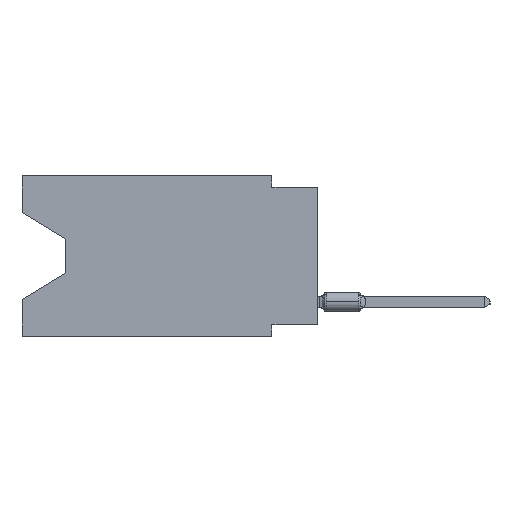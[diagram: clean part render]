
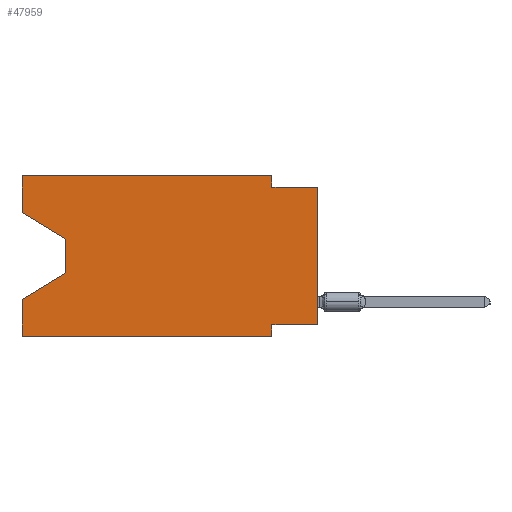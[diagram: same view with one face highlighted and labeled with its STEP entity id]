
A CAD part, left-side view. The second image highlights one B-rep face of the part: STEP entity #47959.
In plain terms, the highlighted planar face has unit normal (-1, 0, 0).
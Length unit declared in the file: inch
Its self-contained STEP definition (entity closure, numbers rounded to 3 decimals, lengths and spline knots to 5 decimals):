
#193 = LINE ( 'NONE', #41502, #43727 ) ;
#1086 = CARTESIAN_POINT ( 'NONE',  ( 0., 0.1, -0.325 ) ) ;
#1662 = EDGE_CURVE ( 'NONE', #44634, #39358, #8237, .T. ) ;
#1699 = ORIENTED_EDGE ( 'NONE', *, *, #1662, .F. ) ;
#5048 = VECTOR ( 'NONE', #38399, 39.37008 ) ;
#6948 = PLANE ( 'NONE',  #66461 ) ;
#7233 = CARTESIAN_POINT ( 'NONE',  ( 0., 0.1, -0.35 ) ) ;
#8237 = LINE ( 'NONE', #35169, #15306 ) ;
#8245 = CARTESIAN_POINT ( 'NONE',  ( 0., 0., 0. ) ) ;
#8708 = CARTESIAN_POINT ( 'NONE',  ( 0., 0.645, -0.08025 ) ) ;
#11009 = DIRECTION ( 'NONE',  ( 0., 0., -1. ) ) ;
#11106 = VERTEX_POINT ( 'NONE', #8708 ) ;
#11544 = DIRECTION ( 'NONE',  ( 0., 0.855, -0.519 ) ) ;
#11688 = VERTEX_POINT ( 'NONE', #55358 ) ;
#12210 = FACE_OUTER_BOUND ( 'NONE', #42204, .T. ) ;
#15266 = DIRECTION ( 'NONE',  ( 0., 0., -1. ) ) ;
#15306 = VECTOR ( 'NONE', #46365, 39.37008 ) ;
#16614 = VERTEX_POINT ( 'NONE', #1086 ) ;
#17595 = VECTOR ( 'NONE', #21850, 39.37008 ) ;
#18417 = LINE ( 'NONE', #8245, #66617 ) ;
#19380 = CARTESIAN_POINT ( 'NONE',  ( 0., 0.1, -0.025 ) ) ;
#20049 = VERTEX_POINT ( 'NONE', #58505 ) ;
#20349 = VERTEX_POINT ( 'NONE', #51467 ) ;
#21512 = CARTESIAN_POINT ( 'NONE',  ( 0., 0.645, 0. ) ) ;
#21850 = DIRECTION ( 'NONE',  ( 0., 0., 1. ) ) ;
#22328 = CARTESIAN_POINT ( 'NONE',  ( 0., 0., -0.325 ) ) ;
#23044 = DIRECTION ( 'NONE',  ( 1., 0., 0. ) ) ;
#23135 = CARTESIAN_POINT ( 'NONE',  ( 0., 0.645, -0.35 ) ) ;
#23706 = EDGE_CURVE ( 'NONE', #39358, #31492, #44220, .T. ) ;
#23986 = CARTESIAN_POINT ( 'NONE',  ( 0., 0.645, -0.08025 ) ) ;
#24188 = ORIENTED_EDGE ( 'NONE', *, *, #49521, .T. ) ;
#24286 = EDGE_CURVE ( 'NONE', #65336, #20349, #50383, .T. ) ;
#24344 = LINE ( 'NONE', #35849, #36367 ) ;
#24945 = ORIENTED_EDGE ( 'NONE', *, *, #31799, .F. ) ;
#27012 = CARTESIAN_POINT ( 'NONE',  ( 0., 0.55, -0.138 ) ) ;
#27184 = EDGE_CURVE ( 'NONE', #20049, #11688, #38129, .T. ) ;
#27426 = ORIENTED_EDGE ( 'NONE', *, *, #64969, .F. ) ;
#27688 = VERTEX_POINT ( 'NONE', #27012 ) ;
#28271 = CARTESIAN_POINT ( 'NONE',  ( 0., 0.645, 0. ) ) ;
#28664 = ORIENTED_EDGE ( 'NONE', *, *, #58988, .T. ) ;
#29293 = VECTOR ( 'NONE', #11544, 39.37008 ) ;
#30680 = ORIENTED_EDGE ( 'NONE', *, *, #48420, .F. ) ;
#31492 = VERTEX_POINT ( 'NONE', #19380 ) ;
#31799 = EDGE_CURVE ( 'NONE', #31492, #53319, #38565, .T. ) ;
#31977 = LINE ( 'NONE', #21512, #17595 ) ;
#32711 = VECTOR ( 'NONE', #43818, 39.37008 ) ;
#32771 = VERTEX_POINT ( 'NONE', #64544 ) ;
#33618 = DIRECTION ( 'NONE',  ( 0., -1., 0. ) ) ;
#33987 = VECTOR ( 'NONE', #65604, 39.37008 ) ;
#34493 = DIRECTION ( 'NONE',  ( 0., 0., 1. ) ) ;
#35124 = CARTESIAN_POINT ( 'NONE',  ( 0., 0.645, 0. ) ) ;
#35169 = CARTESIAN_POINT ( 'NONE',  ( 0., 0.645, 0. ) ) ;
#35849 = CARTESIAN_POINT ( 'NONE',  ( 0., 0.645, 0. ) ) ;
#36367 = VECTOR ( 'NONE', #45674, 39.37008 ) ;
#37210 = ORIENTED_EDGE ( 'NONE', *, *, #23706, .F. ) ;
#37277 = CARTESIAN_POINT ( 'NONE',  ( 0., 0.645, -0.35 ) ) ;
#38129 = LINE ( 'NONE', #64357, #29293 ) ;
#38399 = DIRECTION ( 'NONE',  ( 0., 1., 0. ) ) ;
#38565 = LINE ( 'NONE', #64450, #32711 ) ;
#38654 = ORIENTED_EDGE ( 'NONE', *, *, #56511, .F. ) ;
#39358 = VERTEX_POINT ( 'NONE', #50323 ) ;
#40774 = ORIENTED_EDGE ( 'NONE', *, *, #24286, .T. ) ;
#41502 = CARTESIAN_POINT ( 'NONE',  ( 0., 0.55, -0.138 ) ) ;
#42204 = EDGE_LOOP ( 'NONE', ( #67073, #28664, #67995, #49190, #40774, #38654, #27426, #24188, #24945, #37210, #1699, #30680 ) ) ;
#43727 = VECTOR ( 'NONE', #15266, 39.37008 ) ;
#43818 = DIRECTION ( 'NONE',  ( 0., -1., 0. ) ) ;
#44210 = CARTESIAN_POINT ( 'NONE',  ( 0., 0., -0.025 ) ) ;
#44220 = LINE ( 'NONE', #58909, #61406 ) ;
#44634 = VERTEX_POINT ( 'NONE', #35124 ) ;
#45674 = DIRECTION ( 'NONE',  ( 0., 0., 1. ) ) ;
#46365 = DIRECTION ( 'NONE',  ( 0., -1., 0. ) ) ;
#47026 = EDGE_CURVE ( 'NONE', #11106, #27688, #54436, .T. ) ;
#47959 = ADVANCED_FACE ( 'NONE', ( #12210 ), #6948, .F. ) ;
#48055 = VECTOR ( 'NONE', #33618, 39.37008 ) ;
#48420 = EDGE_CURVE ( 'NONE', #11106, #44634, #24344, .T. ) ;
#48906 = LINE ( 'NONE', #22328, #5048 ) ;
#49190 = ORIENTED_EDGE ( 'NONE', *, *, #67798, .F. ) ;
#49521 = EDGE_CURVE ( 'NONE', #32771, #53319, #18417, .T. ) ;
#49563 = DIRECTION ( 'NONE',  ( 0., 0., -1. ) ) ;
#50323 = CARTESIAN_POINT ( 'NONE',  ( 0., 0.1, 0. ) ) ;
#50383 = LINE ( 'NONE', #23135, #48055 ) ;
#51467 = CARTESIAN_POINT ( 'NONE',  ( 0., 0.1, -0.35 ) ) ;
#53319 = VERTEX_POINT ( 'NONE', #44210 ) ;
#54436 = LINE ( 'NONE', #23986, #33987 ) ;
#55358 = CARTESIAN_POINT ( 'NONE',  ( 0., 0.645, -0.26975 ) ) ;
#56511 = EDGE_CURVE ( 'NONE', #16614, #20349, #60390, .T. ) ;
#58505 = CARTESIAN_POINT ( 'NONE',  ( 0., 0.55, -0.212 ) ) ;
#58909 = CARTESIAN_POINT ( 'NONE',  ( 0., 0.1, 0. ) ) ;
#58988 = EDGE_CURVE ( 'NONE', #27688, #20049, #193, .T. ) ;
#60390 = LINE ( 'NONE', #7233, #63577 ) ;
#61406 = VECTOR ( 'NONE', #11009, 39.37008 ) ;
#63577 = VECTOR ( 'NONE', #49563, 39.37008 ) ;
#64357 = CARTESIAN_POINT ( 'NONE',  ( 0., 0.55, -0.212 ) ) ;
#64450 = CARTESIAN_POINT ( 'NONE',  ( 0., 0., -0.025 ) ) ;
#64544 = CARTESIAN_POINT ( 'NONE',  ( 0., 0., -0.325 ) ) ;
#64969 = EDGE_CURVE ( 'NONE', #32771, #16614, #48906, .T. ) ;
#65336 = VERTEX_POINT ( 'NONE', #37277 ) ;
#65604 = DIRECTION ( 'NONE',  ( 0., -0.855, -0.519 ) ) ;
#65693 = DIRECTION ( 'NONE',  ( 0., 0., -1. ) ) ;
#66461 = AXIS2_PLACEMENT_3D ( 'NONE', #28271, #23044, #65693 ) ;
#66617 = VECTOR ( 'NONE', #34493, 39.37008 ) ;
#67073 = ORIENTED_EDGE ( 'NONE', *, *, #47026, .T. ) ;
#67798 = EDGE_CURVE ( 'NONE', #65336, #11688, #31977, .T. ) ;
#67995 = ORIENTED_EDGE ( 'NONE', *, *, #27184, .T. ) ;
